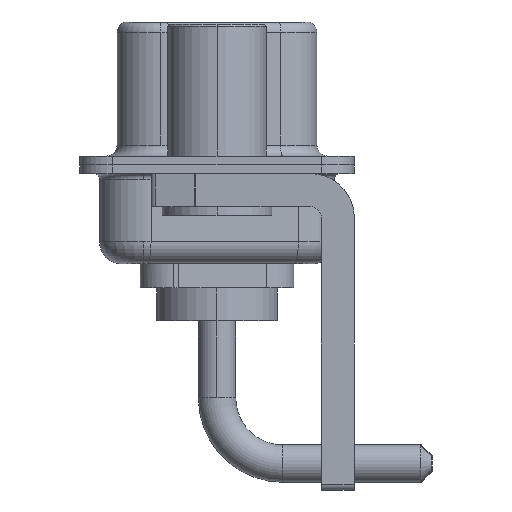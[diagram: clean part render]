
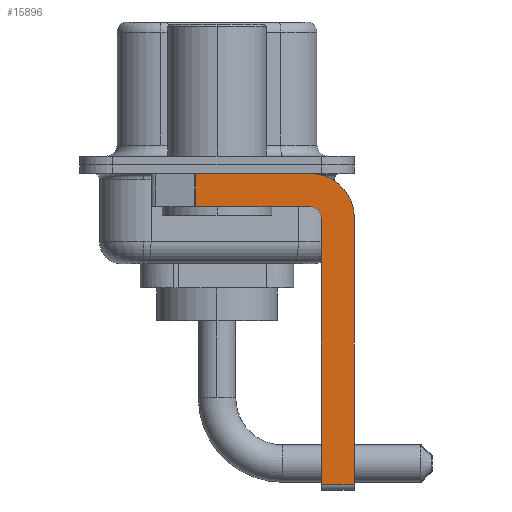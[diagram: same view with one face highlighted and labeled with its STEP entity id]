
A CAD part, left-side view. The second image highlights one B-rep face of the part: STEP entity #15896.
In plain terms, the highlighted planar face has unit normal (-1, 0, 0).
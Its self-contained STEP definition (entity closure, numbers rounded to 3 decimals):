
#208 = VERTEX_POINT ( 'NONE', #16200 ) ;
#243 = VERTEX_POINT ( 'NONE', #7165 ) ;
#253 = VECTOR ( 'NONE', #8409, 1000. ) ;
#1035 = DIRECTION ( 'NONE',  ( 0., -1., 0. ) ) ;
#1185 = AXIS2_PLACEMENT_3D ( 'NONE', #14154, #5121, #9164 ) ;
#1454 = LINE ( 'NONE', #1537, #15679 ) ;
#1537 = CARTESIAN_POINT ( 'NONE',  ( -2.9, 0.978, -1.9 ) ) ;
#1868 = DIRECTION ( 'NONE',  ( 0., -1., 0. ) ) ;
#2133 = DIRECTION ( 'NONE',  ( 0., 0., -1. ) ) ;
#2409 = CARTESIAN_POINT ( 'NONE',  ( -2.9, 3., -0.4 ) ) ;
#3068 = CARTESIAN_POINT ( 'NONE',  ( -2.9, -4.75, -14.8 ) ) ;
#3430 = DIRECTION ( 'NONE',  ( 1., 0., 0. ) ) ;
#3472 = ORIENTED_EDGE ( 'NONE', *, *, #8876, .F. ) ;
#3548 = EDGE_CURVE ( 'NONE', #243, #14368, #12089, .T. ) ;
#3635 = ORIENTED_EDGE ( 'NONE', *, *, #3548, .F. ) ;
#3982 = CARTESIAN_POINT ( 'NONE',  ( -2.9, -4.25, -2.4 ) ) ;
#4150 = DIRECTION ( 'NONE',  ( 0., 1., 0. ) ) ;
#4392 = VERTEX_POINT ( 'NONE', #6281 ) ;
#4411 = ORIENTED_EDGE ( 'NONE', *, *, #15450, .F. ) ;
#4749 = ORIENTED_EDGE ( 'NONE', *, *, #13330, .F. ) ;
#4798 = PLANE ( 'NONE',  #12393 ) ;
#5001 = CIRCLE ( 'NONE', #16438, 0.5 ) ;
#5121 = DIRECTION ( 'NONE',  ( 1., 0., 0. ) ) ;
#5419 = CARTESIAN_POINT ( 'NONE',  ( -2.9, -4.25, -1.9 ) ) ;
#6281 = CARTESIAN_POINT ( 'NONE',  ( -2.9, -6.25, -14.55 ) ) ;
#6358 = VECTOR ( 'NONE', #1035, 1000. ) ;
#6832 = EDGE_CURVE ( 'NONE', #13202, #13277, #12877, .T. ) ;
#6914 = LINE ( 'NONE', #13068, #8573 ) ;
#7165 = CARTESIAN_POINT ( 'NONE',  ( -2.9, -4.75, -14.55 ) ) ;
#7420 = CARTESIAN_POINT ( 'NONE',  ( -2.9, -4.25, -2.4 ) ) ;
#7442 = VECTOR ( 'NONE', #7794, 1000. ) ;
#7507 = FACE_OUTER_BOUND ( 'NONE', #12179, .T. ) ;
#7794 = DIRECTION ( 'NONE',  ( 0., 0., -1. ) ) ;
#7980 = EDGE_CURVE ( 'NONE', #14368, #16242, #5001, .T. ) ;
#8009 = DIRECTION ( 'NONE',  ( 0., 0., -1. ) ) ;
#8409 = DIRECTION ( 'NONE',  ( 0., 0., 1. ) ) ;
#8573 = VECTOR ( 'NONE', #1868, 1000. ) ;
#8717 = CARTESIAN_POINT ( 'NONE',  ( -2.9, 0.978, -1.9 ) ) ;
#8876 = EDGE_CURVE ( 'NONE', #13277, #208, #15615, .T. ) ;
#9098 = VECTOR ( 'NONE', #4150, 1000. ) ;
#9164 = DIRECTION ( 'NONE',  ( 0., 0., -1. ) ) ;
#9229 = DIRECTION ( 'NONE',  ( 0., 0., 1. ) ) ;
#10356 = CARTESIAN_POINT ( 'NONE',  ( -2.9, -4.25, -0.4 ) ) ;
#11106 = ORIENTED_EDGE ( 'NONE', *, *, #15877, .T. ) ;
#11798 = DIRECTION ( 'NONE',  ( -1., 0., 0. ) ) ;
#11922 = ORIENTED_EDGE ( 'NONE', *, *, #6832, .F. ) ;
#12089 = LINE ( 'NONE', #3068, #253 ) ;
#12179 = EDGE_LOOP ( 'NONE', ( #11922, #13458, #4411, #13615, #3635, #11106, #4749, #3472 ) ) ;
#12393 = AXIS2_PLACEMENT_3D ( 'NONE', #7420, #3430, #2133 ) ;
#12877 = LINE ( 'NONE', #2409, #6358 ) ;
#13068 = CARTESIAN_POINT ( 'NONE',  ( -2.9, -4.25, -14.55 ) ) ;
#13202 = VERTEX_POINT ( 'NONE', #16431 ) ;
#13204 = CARTESIAN_POINT ( 'NONE',  ( -2.9, -4.75, -2.4 ) ) ;
#13277 = VERTEX_POINT ( 'NONE', #10356 ) ;
#13330 = EDGE_CURVE ( 'NONE', #208, #4392, #14286, .T. ) ;
#13458 = ORIENTED_EDGE ( 'NONE', *, *, #16540, .T. ) ;
#13615 = ORIENTED_EDGE ( 'NONE', *, *, #7980, .F. ) ;
#14154 = CARTESIAN_POINT ( 'NONE',  ( -2.9, -4.25, -2.4 ) ) ;
#14286 = LINE ( 'NONE', #16842, #7442 ) ;
#14368 = VERTEX_POINT ( 'NONE', #13204 ) ;
#15450 = EDGE_CURVE ( 'NONE', #16242, #15667, #15815, .T. ) ;
#15615 = CIRCLE ( 'NONE', #1185, 2. ) ;
#15667 = VERTEX_POINT ( 'NONE', #8717 ) ;
#15679 = VECTOR ( 'NONE', #8009, 1000. ) ;
#15815 = LINE ( 'NONE', #5419, #9098 ) ;
#15877 = EDGE_CURVE ( 'NONE', #243, #4392, #6914, .T. ) ;
#15896 = ADVANCED_FACE ( 'NONE', ( #7507 ), #4798, .F. ) ;
#16200 = CARTESIAN_POINT ( 'NONE',  ( -2.9, -6.25, -2.4 ) ) ;
#16242 = VERTEX_POINT ( 'NONE', #16403 ) ;
#16403 = CARTESIAN_POINT ( 'NONE',  ( -2.9, -4.25, -1.9 ) ) ;
#16431 = CARTESIAN_POINT ( 'NONE',  ( -2.9, 0.978, -0.4 ) ) ;
#16438 = AXIS2_PLACEMENT_3D ( 'NONE', #3982, #11798, #9229 ) ;
#16540 = EDGE_CURVE ( 'NONE', #13202, #15667, #1454, .T. ) ;
#16842 = CARTESIAN_POINT ( 'NONE',  ( -2.9, -6.25, -2.4 ) ) ;
